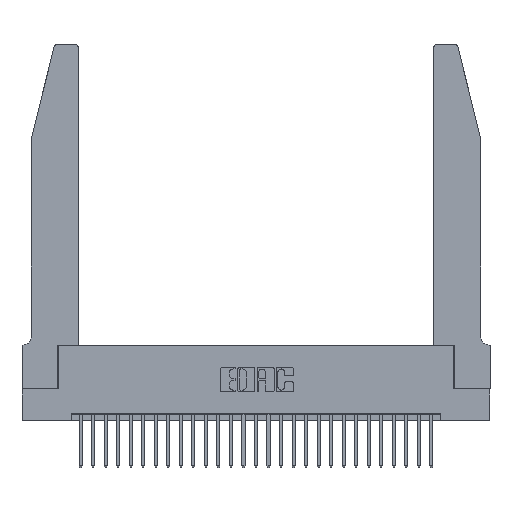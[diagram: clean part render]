
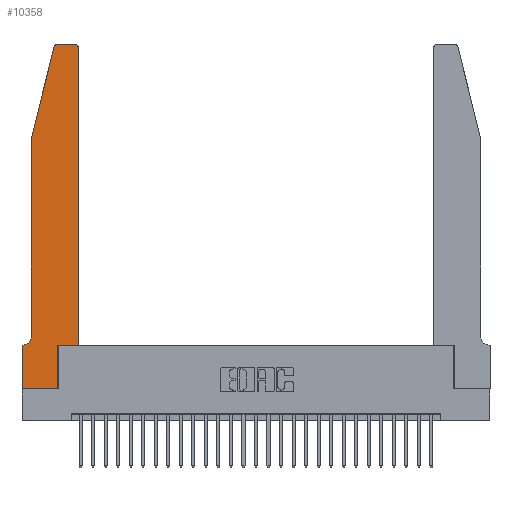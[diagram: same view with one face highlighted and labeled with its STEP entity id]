
A CAD part, top view. The second image highlights one B-rep face of the part: STEP entity #10358.
In plain terms, the highlighted planar face has unit normal (0, 0, 1).
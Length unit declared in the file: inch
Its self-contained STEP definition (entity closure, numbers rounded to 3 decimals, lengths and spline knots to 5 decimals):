
#356 = LINE ( 'NONE', #15964, #17972 ) ;
#498 = CARTESIAN_POINT ( 'NONE',  ( 0., 0., 0.37 ) ) ;
#680 = VECTOR ( 'NONE', #5022, 39.37008 ) ;
#883 = DIRECTION ( 'NONE',  ( 0., 0., 1. ) ) ;
#1043 = LINE ( 'NONE', #17463, #24501 ) ;
#2091 = CIRCLE ( 'NONE', #25592, 0.03 ) ;
#2322 = CARTESIAN_POINT ( 'NONE',  ( 0.2865, 0., 0.37 ) ) ;
#2671 = CARTESIAN_POINT ( 'NONE',  ( 0.4505, 0.35, 0.37 ) ) ;
#2890 = ORIENTED_EDGE ( 'NONE', *, *, #25403, .T. ) ;
#3059 = CARTESIAN_POINT ( 'NONE',  ( 0.0755, 2., 0.37 ) ) ;
#3108 = ORIENTED_EDGE ( 'NONE', *, *, #24646, .T. ) ;
#3142 = VERTEX_POINT ( 'NONE', #2322 ) ;
#3628 = ORIENTED_EDGE ( 'NONE', *, *, #5056, .T. ) ;
#3815 = ORIENTED_EDGE ( 'NONE', *, *, #22639, .T. ) ;
#4099 = VERTEX_POINT ( 'NONE', #10488 ) ;
#4546 = ORIENTED_EDGE ( 'NONE', *, *, #24602, .T. ) ;
#4663 = CIRCLE ( 'NONE', #18740, 0.07 ) ;
#5022 = DIRECTION ( 'NONE',  ( 0., 1., 0. ) ) ;
#5056 = EDGE_CURVE ( 'NONE', #20528, #19756, #5288, .T. ) ;
#5071 = DIRECTION ( 'NONE',  ( 1., 0., 0. ) ) ;
#5187 = EDGE_LOOP ( 'NONE', ( #3628, #4546, #18811, #3815, #17950, #8091, #29304, #3108, #22348, #25487, #26415, #2890 ) ) ;
#5288 = LINE ( 'NONE', #6720, #10734 ) ;
#5665 = DIRECTION ( 'NONE',  ( 0., 1., 0. ) ) ;
#6720 = CARTESIAN_POINT ( 'NONE',  ( 0.2605, 2.75, 0.37 ) ) ;
#7186 = CARTESIAN_POINT ( 'NONE',  ( 0.4205, 2.75, 0.37 ) ) ;
#7302 = EDGE_CURVE ( 'NONE', #3142, #17784, #16574, .T. ) ;
#7324 = DIRECTION ( 'NONE',  ( 0., 0., 1. ) ) ;
#8091 = ORIENTED_EDGE ( 'NONE', *, *, #27598, .T. ) ;
#8210 = VERTEX_POINT ( 'NONE', #20289 ) ;
#8231 = LINE ( 'NONE', #13764, #19551 ) ;
#9517 = EDGE_CURVE ( 'NONE', #10406, #13415, #13717, .T. ) ;
#10142 = DIRECTION ( 'NONE',  ( 0., 0., 1. ) ) ;
#10163 = LINE ( 'NONE', #11652, #15462 ) ;
#10358 = ADVANCED_FACE ( 'NONE', ( #20994 ), #14606, .T. ) ;
#10406 = VERTEX_POINT ( 'NONE', #19296 ) ;
#10488 = CARTESIAN_POINT ( 'NONE',  ( 0.25487, 2.72718, 0.37 ) ) ;
#10601 = VECTOR ( 'NONE', #5665, 39.37008 ) ;
#10734 = VECTOR ( 'NONE', #20298, 39.37008 ) ;
#11652 = CARTESIAN_POINT ( 'NONE',  ( 0.4505, 0.35, 0.37 ) ) ;
#12229 = LINE ( 'NONE', #23167, #24089 ) ;
#12642 = DIRECTION ( 'NONE',  ( 1., 0., 0. ) ) ;
#13034 = DIRECTION ( 'NONE',  ( 0., 0., -1. ) ) ;
#13061 = DIRECTION ( 'NONE',  ( 0., -1., 0. ) ) ;
#13271 = LINE ( 'NONE', #22056, #18545 ) ;
#13415 = VERTEX_POINT ( 'NONE', #28265 ) ;
#13503 = AXIS2_PLACEMENT_3D ( 'NONE', #14705, #883, #16957 ) ;
#13717 = LINE ( 'NONE', #2671, #680 ) ;
#13764 = CARTESIAN_POINT ( 'NONE',  ( 0.0755, 2., 0.37 ) ) ;
#14329 = CARTESIAN_POINT ( 'NONE',  ( 0., 0.35, 0.37 ) ) ;
#14606 = PLANE ( 'NONE',  #26310 ) ;
#14705 = CARTESIAN_POINT ( 'NONE',  ( 0.4205, 2.72, 0.37 ) ) ;
#14889 = VERTEX_POINT ( 'NONE', #14329 ) ;
#15462 = VECTOR ( 'NONE', #12642, 39.37008 ) ;
#15899 = CARTESIAN_POINT ( 'NONE',  ( 0.0055, 0.35, 0.37 ) ) ;
#15964 = CARTESIAN_POINT ( 'NONE',  ( 0.0755, 2., 0.37 ) ) ;
#15971 = CARTESIAN_POINT ( 'NONE',  ( 0.284, 2.75, 0.37 ) ) ;
#16016 = DIRECTION ( 'NONE',  ( -0.239, -0.971, 0. ) ) ;
#16574 = LINE ( 'NONE', #19205, #10601 ) ;
#16815 = EDGE_CURVE ( 'NONE', #4099, #24072, #8231, .T. ) ;
#16957 = DIRECTION ( 'NONE',  ( 1., 0., 0. ) ) ;
#17463 = CARTESIAN_POINT ( 'NONE',  ( 0.0755, 0.35, 0.37 ) ) ;
#17736 = CARTESIAN_POINT ( 'NONE',  ( 0.2865, 0.35, 0.37 ) ) ;
#17784 = VERTEX_POINT ( 'NONE', #17736 ) ;
#17950 = ORIENTED_EDGE ( 'NONE', *, *, #24274, .T. ) ;
#17972 = VECTOR ( 'NONE', #20463, 39.37008 ) ;
#18545 = VECTOR ( 'NONE', #13061, 39.37008 ) ;
#18740 = AXIS2_PLACEMENT_3D ( 'NONE', #26356, #13034, #28574 ) ;
#18811 = ORIENTED_EDGE ( 'NONE', *, *, #16815, .T. ) ;
#19205 = CARTESIAN_POINT ( 'NONE',  ( 0.2865, 0.35, 0.37 ) ) ;
#19296 = CARTESIAN_POINT ( 'NONE',  ( 0.4505, 0.35, 0.37 ) ) ;
#19551 = VECTOR ( 'NONE', #16016, 39.37008 ) ;
#19756 = VERTEX_POINT ( 'NONE', #15971 ) ;
#20289 = CARTESIAN_POINT ( 'NONE',  ( 0.0755, 0.42, 0.37 ) ) ;
#20298 = DIRECTION ( 'NONE',  ( -1., 0., 0. ) ) ;
#20463 = DIRECTION ( 'NONE',  ( 0., -1., 0. ) ) ;
#20528 = VERTEX_POINT ( 'NONE', #7186 ) ;
#20848 = CARTESIAN_POINT ( 'NONE',  ( 0.284, 2.72, 0.37 ) ) ;
#20994 = FACE_OUTER_BOUND ( 'NONE', #5187, .T. ) ;
#21059 = VERTEX_POINT ( 'NONE', #15899 ) ;
#21932 = DIRECTION ( 'NONE',  ( -1., 0., 0. ) ) ;
#22056 = CARTESIAN_POINT ( 'NONE',  ( 0., 0., 0.37 ) ) ;
#22348 = ORIENTED_EDGE ( 'NONE', *, *, #7302, .T. ) ;
#22639 = EDGE_CURVE ( 'NONE', #24072, #8210, #356, .T. ) ;
#23066 = DIRECTION ( 'NONE',  ( 1., 0., 0. ) ) ;
#23167 = CARTESIAN_POINT ( 'NONE',  ( 0., 0., 0.37 ) ) ;
#23548 = CARTESIAN_POINT ( 'NONE',  ( 0., 0.35, 0.37 ) ) ;
#23686 = CIRCLE ( 'NONE', #13503, 0.03 ) ;
#24072 = VERTEX_POINT ( 'NONE', #3059 ) ;
#24089 = VECTOR ( 'NONE', #5071, 39.37008 ) ;
#24274 = EDGE_CURVE ( 'NONE', #8210, #21059, #4663, .T. ) ;
#24501 = VECTOR ( 'NONE', #21932, 39.37008 ) ;
#24602 = EDGE_CURVE ( 'NONE', #19756, #4099, #2091, .T. ) ;
#24646 = EDGE_CURVE ( 'NONE', #29230, #3142, #12229, .T. ) ;
#25403 = EDGE_CURVE ( 'NONE', #13415, #20528, #23686, .T. ) ;
#25487 = ORIENTED_EDGE ( 'NONE', *, *, #27533, .T. ) ;
#25592 = AXIS2_PLACEMENT_3D ( 'NONE', #20848, #7324, #23066 ) ;
#25753 = DIRECTION ( 'NONE',  ( 1., 0., 0. ) ) ;
#26310 = AXIS2_PLACEMENT_3D ( 'NONE', #23548, #10142, #25753 ) ;
#26356 = CARTESIAN_POINT ( 'NONE',  ( 0.0055, 0.42, 0.37 ) ) ;
#26415 = ORIENTED_EDGE ( 'NONE', *, *, #9517, .T. ) ;
#27533 = EDGE_CURVE ( 'NONE', #17784, #10406, #10163, .T. ) ;
#27598 = EDGE_CURVE ( 'NONE', #21059, #14889, #1043, .T. ) ;
#28265 = CARTESIAN_POINT ( 'NONE',  ( 0.4505, 2.72, 0.37 ) ) ;
#28574 = DIRECTION ( 'NONE',  ( -1., 0., 0. ) ) ;
#28971 = EDGE_CURVE ( 'NONE', #14889, #29230, #13271, .T. ) ;
#29230 = VERTEX_POINT ( 'NONE', #498 ) ;
#29304 = ORIENTED_EDGE ( 'NONE', *, *, #28971, .T. ) ;
